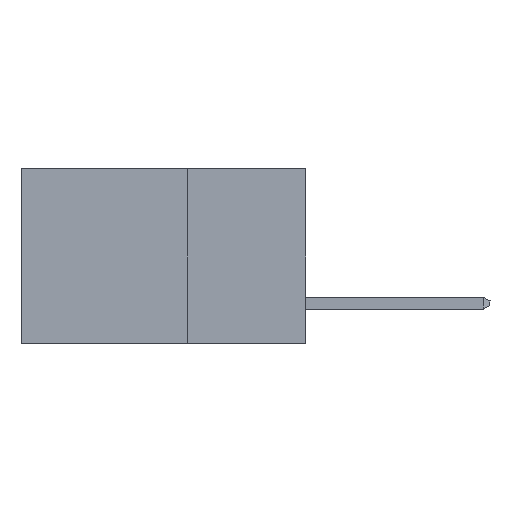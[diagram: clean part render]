
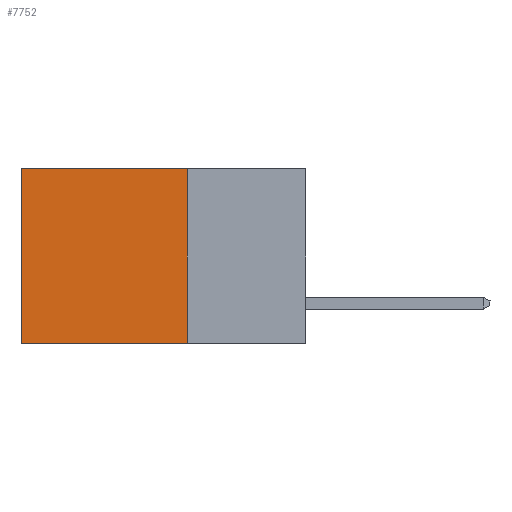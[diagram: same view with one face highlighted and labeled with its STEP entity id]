
A CAD part, left-side view. The second image highlights one B-rep face of the part: STEP entity #7752.
In plain terms, the highlighted planar face has unit normal (-1, 0, 0).
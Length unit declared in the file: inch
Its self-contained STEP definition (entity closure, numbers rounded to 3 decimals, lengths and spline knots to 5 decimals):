
#805 = VECTOR ( 'NONE', #3954, 39.37008 ) ;
#809 = CARTESIAN_POINT ( 'NONE',  ( 0.2615, 0.25, 0. ) ) ;
#1130 = DIRECTION ( 'NONE',  ( 1., 0., 0. ) ) ;
#1142 = ORIENTED_EDGE ( 'NONE', *, *, #4326, .T. ) ;
#1178 = EDGE_CURVE ( 'NONE', #9554, #10592, #5898, .T. ) ;
#1544 = VECTOR ( 'NONE', #4184, 39.37008 ) ;
#2076 = VERTEX_POINT ( 'NONE', #3326 ) ;
#2530 = LINE ( 'NONE', #809, #1544 ) ;
#2602 = VECTOR ( 'NONE', #8561, 39.37008 ) ;
#2947 = FACE_OUTER_BOUND ( 'NONE', #7853, .T. ) ;
#3326 = CARTESIAN_POINT ( 'NONE',  ( 0.2615, 0.25, 0. ) ) ;
#3688 = AXIS2_PLACEMENT_3D ( 'NONE', #6219, #1130, #4482 ) ;
#3811 = EDGE_CURVE ( 'NONE', #4488, #10592, #4802, .T. ) ;
#3954 = DIRECTION ( 'NONE',  ( 0., 1., 0. ) ) ;
#4184 = DIRECTION ( 'NONE',  ( 0., 1., 0. ) ) ;
#4326 = EDGE_CURVE ( 'NONE', #2076, #9554, #2530, .T. ) ;
#4328 = CARTESIAN_POINT ( 'NONE',  ( 0.2615, 0.6, -0.37 ) ) ;
#4482 = DIRECTION ( 'NONE',  ( 0., 0., -1. ) ) ;
#4488 = VERTEX_POINT ( 'NONE', #5515 ) ;
#4802 = LINE ( 'NONE', #8004, #805 ) ;
#4986 = EDGE_CURVE ( 'NONE', #2076, #4488, #6115, .T. ) ;
#5295 = CARTESIAN_POINT ( 'NONE',  ( 0.2615, 0.25, -0.37 ) ) ;
#5515 = CARTESIAN_POINT ( 'NONE',  ( 0.2615, 0.25, -0.37 ) ) ;
#5887 = VECTOR ( 'NONE', #8610, 39.37008 ) ;
#5898 = LINE ( 'NONE', #4328, #2602 ) ;
#6115 = LINE ( 'NONE', #5295, #5887 ) ;
#6219 = CARTESIAN_POINT ( 'NONE',  ( 0.2615, 0.25, -0.37 ) ) ;
#6719 = CARTESIAN_POINT ( 'NONE',  ( 0.2615, 0.6, -0.37 ) ) ;
#7686 = ORIENTED_EDGE ( 'NONE', *, *, #1178, .T. ) ;
#7752 = ADVANCED_FACE ( 'NONE', ( #2947 ), #9421, .F. ) ;
#7853 = EDGE_LOOP ( 'NONE', ( #7686, #9592, #10196, #1142 ) ) ;
#7914 = CARTESIAN_POINT ( 'NONE',  ( 0.2615, 0.6, 0. ) ) ;
#8004 = CARTESIAN_POINT ( 'NONE',  ( 0.2615, 0.25, -0.37 ) ) ;
#8561 = DIRECTION ( 'NONE',  ( 0., 0., -1. ) ) ;
#8610 = DIRECTION ( 'NONE',  ( 0., 0., -1. ) ) ;
#9421 = PLANE ( 'NONE',  #3688 ) ;
#9554 = VERTEX_POINT ( 'NONE', #7914 ) ;
#9592 = ORIENTED_EDGE ( 'NONE', *, *, #3811, .F. ) ;
#10196 = ORIENTED_EDGE ( 'NONE', *, *, #4986, .F. ) ;
#10592 = VERTEX_POINT ( 'NONE', #6719 ) ;
